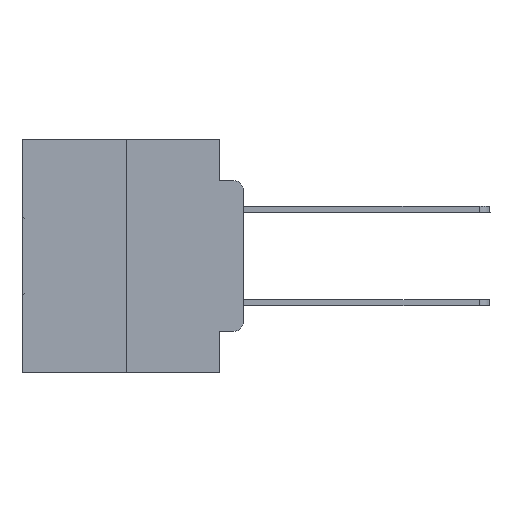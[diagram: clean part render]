
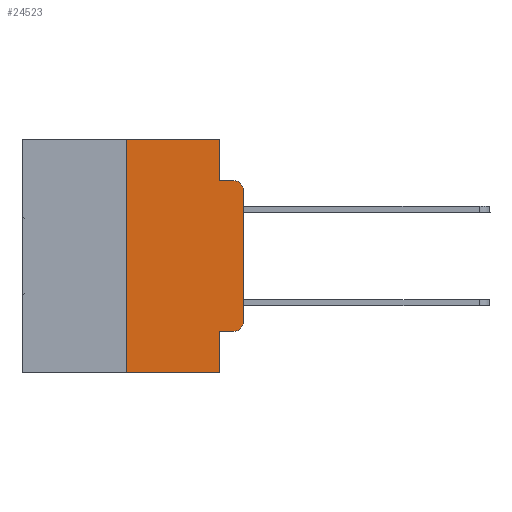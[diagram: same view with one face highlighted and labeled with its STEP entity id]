
A CAD part, left-side view. The second image highlights one B-rep face of the part: STEP entity #24523.
In plain terms, the highlighted planar face has unit normal (-1, 0, 0).
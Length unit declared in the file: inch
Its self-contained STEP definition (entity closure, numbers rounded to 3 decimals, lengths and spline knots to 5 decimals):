
#72 = VECTOR ( 'NONE', #27277, 39.37008 ) ;
#121 = VECTOR ( 'NONE', #28341, 39.37008 ) ;
#407 = EDGE_CURVE ( 'NONE', #23124, #26831, #15386, .T. ) ;
#1066 = VERTEX_POINT ( 'NONE', #26468 ) ;
#1144 = ORIENTED_EDGE ( 'NONE', *, *, #19156, .F. ) ;
#1503 = VECTOR ( 'NONE', #1574, 39.37008 ) ;
#1574 = DIRECTION ( 'NONE',  ( 0., -1., 0. ) ) ;
#3039 = VERTEX_POINT ( 'NONE', #5616 ) ;
#3141 = CARTESIAN_POINT ( 'NONE',  ( 0., 0.051, -0.0885 ) ) ;
#3447 = ORIENTED_EDGE ( 'NONE', *, *, #32039, .F. ) ;
#3729 = DIRECTION ( 'NONE',  ( 0., 0., -1. ) ) ;
#3966 = LINE ( 'NONE', #19412, #32529 ) ;
#4251 = CIRCLE ( 'NONE', #18755, 0.02 ) ;
#4295 = EDGE_CURVE ( 'NONE', #25984, #6041, #13878, .T. ) ;
#4588 = LINE ( 'NONE', #20351, #13911 ) ;
#5088 = DIRECTION ( 'NONE',  ( 0., 0., 1. ) ) ;
#5100 = CARTESIAN_POINT ( 'NONE',  ( 0., 0.051, -0.5 ) ) ;
#5133 = ORIENTED_EDGE ( 'NONE', *, *, #8454, .T. ) ;
#5211 = CARTESIAN_POINT ( 'NONE',  ( 0., 0.02, -0.0885 ) ) ;
#5584 = FACE_OUTER_BOUND ( 'NONE', #17868, .T. ) ;
#5616 = CARTESIAN_POINT ( 'NONE',  ( 0., 0.051, -0.4115 ) ) ;
#6030 = CARTESIAN_POINT ( 'NONE',  ( 0., 0.473, 0. ) ) ;
#6041 = VERTEX_POINT ( 'NONE', #5211 ) ;
#6474 = ORIENTED_EDGE ( 'NONE', *, *, #23265, .F. ) ;
#6730 = CARTESIAN_POINT ( 'NONE',  ( 0., 0.051, 0. ) ) ;
#7005 = LINE ( 'NONE', #21779, #72 ) ;
#7657 = DIRECTION ( 'NONE',  ( -1., 0., 0. ) ) ;
#7715 = CARTESIAN_POINT ( 'NONE',  ( 0., 0.051, 0. ) ) ;
#8279 = DIRECTION ( 'NONE',  ( 0., 0., -1. ) ) ;
#8320 = CARTESIAN_POINT ( 'NONE',  ( 0., 0.02, -0.1085 ) ) ;
#8454 = EDGE_CURVE ( 'NONE', #10986, #25984, #4588, .T. ) ;
#8839 = ORIENTED_EDGE ( 'NONE', *, *, #407, .T. ) ;
#10986 = VERTEX_POINT ( 'NONE', #28530 ) ;
#11058 = DIRECTION ( 'NONE',  ( 0., 0., 1. ) ) ;
#12550 = ORIENTED_EDGE ( 'NONE', *, *, #18367, .F. ) ;
#13878 = CIRCLE ( 'NONE', #27196, 0.02 ) ;
#13911 = VECTOR ( 'NONE', #5088, 39.37008 ) ;
#14350 = AXIS2_PLACEMENT_3D ( 'NONE', #28896, #23701, #8279 ) ;
#15386 = LINE ( 'NONE', #25569, #18070 ) ;
#16894 = LINE ( 'NONE', #18918, #1503 ) ;
#17868 = EDGE_LOOP ( 'NONE', ( #5133, #23090, #12550, #3447, #1144, #32301, #8839, #6474, #20409, #22022 ) ) ;
#18070 = VECTOR ( 'NONE', #18080, 39.37008 ) ;
#18080 = DIRECTION ( 'NONE',  ( 0., -1., 0. ) ) ;
#18085 = DIRECTION ( 'NONE',  ( 0., 0., -1. ) ) ;
#18359 = CARTESIAN_POINT ( 'NONE',  ( 0., 0.25, -0.5 ) ) ;
#18367 = EDGE_CURVE ( 'NONE', #20757, #6041, #16894, .T. ) ;
#18755 = AXIS2_PLACEMENT_3D ( 'NONE', #28731, #23872, #3729 ) ;
#18893 = VERTEX_POINT ( 'NONE', #29865 ) ;
#18918 = CARTESIAN_POINT ( 'NONE',  ( 0., 0.051, -0.0885 ) ) ;
#18927 = LINE ( 'NONE', #29777, #25857 ) ;
#19013 = LINE ( 'NONE', #6730, #33027 ) ;
#19156 = EDGE_CURVE ( 'NONE', #18893, #27681, #29011, .T. ) ;
#19412 = CARTESIAN_POINT ( 'NONE',  ( 0., 0.25, 0. ) ) ;
#19815 = EDGE_CURVE ( 'NONE', #3039, #1066, #18927, .T. ) ;
#20351 = CARTESIAN_POINT ( 'NONE',  ( 0., 0., 0. ) ) ;
#20409 = ORIENTED_EDGE ( 'NONE', *, *, #19815, .T. ) ;
#20757 = VERTEX_POINT ( 'NONE', #3141 ) ;
#21779 = CARTESIAN_POINT ( 'NONE',  ( 0., 0.051, 0. ) ) ;
#21847 = CARTESIAN_POINT ( 'NONE',  ( 0., 0., -0.1085 ) ) ;
#22022 = ORIENTED_EDGE ( 'NONE', *, *, #28307, .T. ) ;
#23090 = ORIENTED_EDGE ( 'NONE', *, *, #4295, .T. ) ;
#23124 = VERTEX_POINT ( 'NONE', #18359 ) ;
#23212 = PLANE ( 'NONE',  #14350 ) ;
#23265 = EDGE_CURVE ( 'NONE', #3039, #26831, #19013, .T. ) ;
#23701 = DIRECTION ( 'NONE',  ( 1., 0., 0. ) ) ;
#23872 = DIRECTION ( 'NONE',  ( -1., 0., 0. ) ) ;
#24173 = DIRECTION ( 'NONE',  ( 0., 0., -1. ) ) ;
#24523 = ADVANCED_FACE ( 'NONE', ( #5584 ), #23212, .F. ) ;
#25473 = EDGE_CURVE ( 'NONE', #23124, #18893, #3966, .T. ) ;
#25569 = CARTESIAN_POINT ( 'NONE',  ( 0., 0.473, -0.5 ) ) ;
#25857 = VECTOR ( 'NONE', #27077, 39.37008 ) ;
#25984 = VERTEX_POINT ( 'NONE', #21847 ) ;
#26468 = CARTESIAN_POINT ( 'NONE',  ( 0., 0.02, -0.4115 ) ) ;
#26831 = VERTEX_POINT ( 'NONE', #5100 ) ;
#27077 = DIRECTION ( 'NONE',  ( 0., -1., 0. ) ) ;
#27196 = AXIS2_PLACEMENT_3D ( 'NONE', #8320, #7657, #18085 ) ;
#27277 = DIRECTION ( 'NONE',  ( 0., 0., -1. ) ) ;
#27681 = VERTEX_POINT ( 'NONE', #7715 ) ;
#28307 = EDGE_CURVE ( 'NONE', #1066, #10986, #4251, .T. ) ;
#28341 = DIRECTION ( 'NONE',  ( 0., -1., 0. ) ) ;
#28530 = CARTESIAN_POINT ( 'NONE',  ( 0., 0., -0.3915 ) ) ;
#28731 = CARTESIAN_POINT ( 'NONE',  ( 0., 0.02, -0.3915 ) ) ;
#28896 = CARTESIAN_POINT ( 'NONE',  ( 0., 0.473, 0. ) ) ;
#29011 = LINE ( 'NONE', #6030, #121 ) ;
#29777 = CARTESIAN_POINT ( 'NONE',  ( 0., 0.051, -0.4115 ) ) ;
#29865 = CARTESIAN_POINT ( 'NONE',  ( 0., 0.25, 0. ) ) ;
#32039 = EDGE_CURVE ( 'NONE', #27681, #20757, #7005, .T. ) ;
#32301 = ORIENTED_EDGE ( 'NONE', *, *, #25473, .F. ) ;
#32529 = VECTOR ( 'NONE', #11058, 39.37008 ) ;
#33027 = VECTOR ( 'NONE', #24173, 39.37008 ) ;
